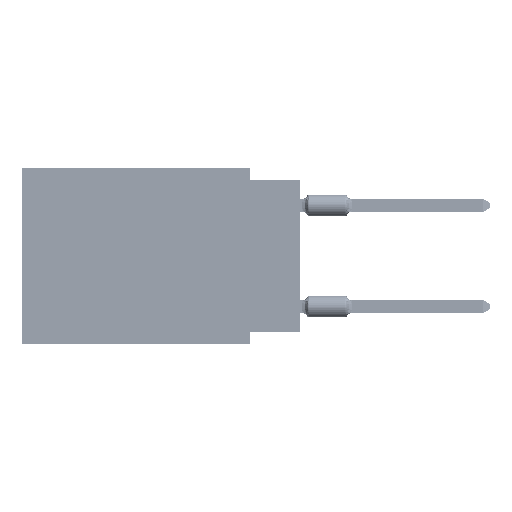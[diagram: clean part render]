
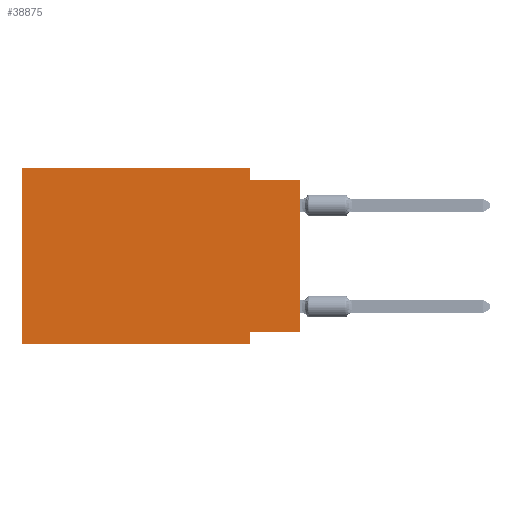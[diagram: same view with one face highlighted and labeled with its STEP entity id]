
A CAD part, left-side view. The second image highlights one B-rep face of the part: STEP entity #38875.
In plain terms, the highlighted planar face has unit normal (-1, 0, 0).
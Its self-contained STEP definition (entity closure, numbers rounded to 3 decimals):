
#1849 = ORIENTED_EDGE ( 'NONE', *, *, #40455, .F. ) ;
#10875 = ORIENTED_EDGE ( 'NONE', *, *, #71410, .F. ) ;
#16062 = DIRECTION ( 'NONE',  ( 0., 1., 0. ) ) ;
#17682 = EDGE_LOOP ( 'NONE', ( #41442, #33785, #53566, #1849, #26095, #84469, #75840, #10875 ) ) ;
#18911 = DIRECTION ( 'NONE',  ( 0., 0., 1. ) ) ;
#20512 = VERTEX_POINT ( 'NONE', #56992 ) ;
#24474 = VECTOR ( 'NONE', #106166, 1000. ) ;
#26086 = CARTESIAN_POINT ( 'NONE',  ( 0., 13.97, -8.89 ) ) ;
#26095 = ORIENTED_EDGE ( 'NONE', *, *, #105979, .F. ) ;
#26535 = CARTESIAN_POINT ( 'NONE',  ( 0., 2.54, -0.635 ) ) ;
#27890 = DIRECTION ( 'NONE',  ( 0., -1., 0. ) ) ;
#30436 = CARTESIAN_POINT ( 'NONE',  ( 0., 2.54, -8.89 ) ) ;
#30897 = LINE ( 'NONE', #32077, #36025 ) ;
#32033 = DIRECTION ( 'NONE',  ( 1., 0., 0. ) ) ;
#32077 = CARTESIAN_POINT ( 'NONE',  ( 0., 0., -0.635 ) ) ;
#33785 = ORIENTED_EDGE ( 'NONE', *, *, #78904, .F. ) ;
#34095 = CARTESIAN_POINT ( 'NONE',  ( 0., 2.54, -8.255 ) ) ;
#36025 = VECTOR ( 'NONE', #58596, 1000. ) ;
#38875 = ADVANCED_FACE ( 'NONE', ( #41270 ), #50525, .F. ) ;
#40455 = EDGE_CURVE ( 'NONE', #20512, #43002, #48944, .T. ) ;
#41270 = FACE_OUTER_BOUND ( 'NONE', #17682, .T. ) ;
#41442 = ORIENTED_EDGE ( 'NONE', *, *, #78121, .T. ) ;
#43002 = VERTEX_POINT ( 'NONE', #106354 ) ;
#43856 = VERTEX_POINT ( 'NONE', #60893 ) ;
#45598 = CARTESIAN_POINT ( 'NONE',  ( 0., 0., -8.255 ) ) ;
#45754 = VECTOR ( 'NONE', #109499, 1000. ) ;
#45838 = AXIS2_PLACEMENT_3D ( 'NONE', #116379, #32033, #68382 ) ;
#47061 = VECTOR ( 'NONE', #16062, 1000. ) ;
#48944 = LINE ( 'NONE', #115421, #24474 ) ;
#50525 = PLANE ( 'NONE',  #45838 ) ;
#51345 = CARTESIAN_POINT ( 'NONE',  ( 0., 13.97, -8.89 ) ) ;
#52836 = DIRECTION ( 'NONE',  ( 0., 0., -1. ) ) ;
#53566 = ORIENTED_EDGE ( 'NONE', *, *, #55421, .F. ) ;
#55421 = EDGE_CURVE ( 'NONE', #43002, #61356, #82983, .T. ) ;
#56992 = CARTESIAN_POINT ( 'NONE',  ( 0., 13.97, 0. ) ) ;
#57471 = VERTEX_POINT ( 'NONE', #34095 ) ;
#58596 = DIRECTION ( 'NONE',  ( 0., -1., 0. ) ) ;
#60893 = CARTESIAN_POINT ( 'NONE',  ( 0., 0., -0.635 ) ) ;
#61356 = VERTEX_POINT ( 'NONE', #26535 ) ;
#67554 = VERTEX_POINT ( 'NONE', #30436 ) ;
#68382 = DIRECTION ( 'NONE',  ( 0., 0., -1. ) ) ;
#68708 = CARTESIAN_POINT ( 'NONE',  ( 0., 0., 0. ) ) ;
#71410 = EDGE_CURVE ( 'NONE', #76194, #57471, #80717, .T. ) ;
#72072 = VERTEX_POINT ( 'NONE', #51345 ) ;
#72158 = EDGE_CURVE ( 'NONE', #72072, #67554, #72859, .T. ) ;
#72859 = LINE ( 'NONE', #26086, #88255 ) ;
#75840 = ORIENTED_EDGE ( 'NONE', *, *, #96077, .F. ) ;
#76194 = VERTEX_POINT ( 'NONE', #86290 ) ;
#78121 = EDGE_CURVE ( 'NONE', #76194, #43856, #115533, .T. ) ;
#78904 = EDGE_CURVE ( 'NONE', #61356, #43856, #30897, .T. ) ;
#80717 = LINE ( 'NONE', #45598, #47061 ) ;
#82450 = CARTESIAN_POINT ( 'NONE',  ( 0., 13.97, 0. ) ) ;
#82983 = LINE ( 'NONE', #93418, #45754 ) ;
#83012 = VECTOR ( 'NONE', #52836, 1000. ) ;
#84469 = ORIENTED_EDGE ( 'NONE', *, *, #72158, .T. ) ;
#86290 = CARTESIAN_POINT ( 'NONE',  ( 0., 0., -8.255 ) ) ;
#88255 = VECTOR ( 'NONE', #27890, 1000. ) ;
#89771 = LINE ( 'NONE', #99001, #83012 ) ;
#91046 = DIRECTION ( 'NONE',  ( 0., 0., 1. ) ) ;
#93418 = CARTESIAN_POINT ( 'NONE',  ( 0., 2.54, 0. ) ) ;
#96077 = EDGE_CURVE ( 'NONE', #57471, #67554, #89771, .T. ) ;
#99001 = CARTESIAN_POINT ( 'NONE',  ( 0., 2.54, -8.89 ) ) ;
#100515 = VECTOR ( 'NONE', #91046, 1000. ) ;
#105979 = EDGE_CURVE ( 'NONE', #72072, #20512, #120614, .T. ) ;
#106166 = DIRECTION ( 'NONE',  ( 0., -1., 0. ) ) ;
#106354 = CARTESIAN_POINT ( 'NONE',  ( 0., 2.54, 0. ) ) ;
#109499 = DIRECTION ( 'NONE',  ( 0., 0., -1. ) ) ;
#115421 = CARTESIAN_POINT ( 'NONE',  ( 0., 13.97, 0. ) ) ;
#115533 = LINE ( 'NONE', #68708, #116729 ) ;
#116379 = CARTESIAN_POINT ( 'NONE',  ( 0., 13.97, 0. ) ) ;
#116729 = VECTOR ( 'NONE', #18911, 1000. ) ;
#120614 = LINE ( 'NONE', #82450, #100515 ) ;
